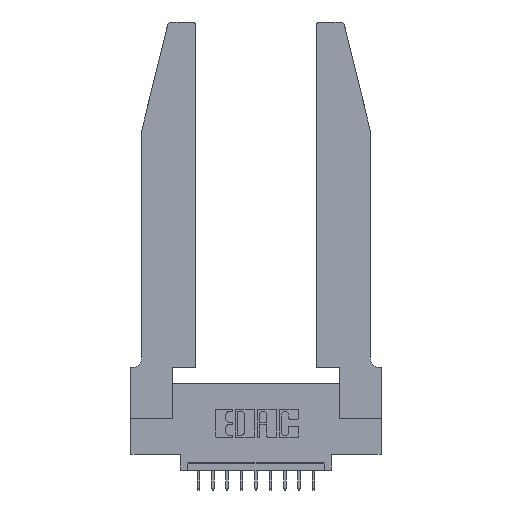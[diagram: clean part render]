
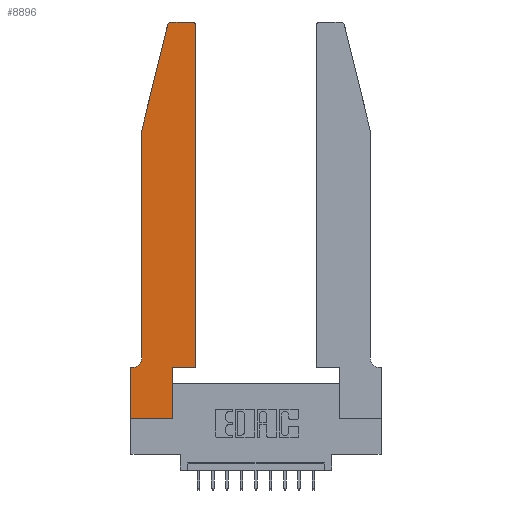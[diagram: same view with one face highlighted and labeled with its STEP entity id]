
A CAD part, top view. The second image highlights one B-rep face of the part: STEP entity #8896.
In plain terms, the highlighted planar face has unit normal (0, 0, 1).
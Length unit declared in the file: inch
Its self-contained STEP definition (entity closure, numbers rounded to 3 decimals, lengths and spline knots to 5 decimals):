
#76 = ORIENTED_EDGE ( 'NONE', *, *, #6097, .T. ) ;
#181 = CARTESIAN_POINT ( 'NONE',  ( 0., 0.35, 0.37 ) ) ;
#246 = EDGE_CURVE ( 'NONE', #8992, #305, #4880, .T. ) ;
#305 = VERTEX_POINT ( 'NONE', #7444 ) ;
#325 = VERTEX_POINT ( 'NONE', #1427 ) ;
#419 = VECTOR ( 'NONE', #12513, 39.37008 ) ;
#554 = CARTESIAN_POINT ( 'NONE',  ( 0.4505, 0.35, 0.37 ) ) ;
#575 = FACE_OUTER_BOUND ( 'NONE', #12629, .T. ) ;
#639 = ORIENTED_EDGE ( 'NONE', *, *, #1111, .T. ) ;
#786 = DIRECTION ( 'NONE',  ( 1., 0., 0. ) ) ;
#902 = VECTOR ( 'NONE', #5218, 39.37008 ) ;
#1111 = EDGE_CURVE ( 'NONE', #7310, #5569, #7624, .T. ) ;
#1407 = PLANE ( 'NONE',  #7855 ) ;
#1427 = CARTESIAN_POINT ( 'NONE',  ( 0., 0., 0.37 ) ) ;
#1849 = CARTESIAN_POINT ( 'NONE',  ( 0.2865, 0., 0.37 ) ) ;
#1931 = VERTEX_POINT ( 'NONE', #10022 ) ;
#2190 = CARTESIAN_POINT ( 'NONE',  ( 0.0755, 2., 0.37 ) ) ;
#2674 = VERTEX_POINT ( 'NONE', #11785 ) ;
#2715 = DIRECTION ( 'NONE',  ( 0., -1., 0. ) ) ;
#2745 = DIRECTION ( 'NONE',  ( 0., 1., 0. ) ) ;
#2868 = VECTOR ( 'NONE', #3057, 39.37008 ) ;
#3057 = DIRECTION ( 'NONE',  ( 0., -1., 0. ) ) ;
#3365 = EDGE_CURVE ( 'NONE', #1931, #7589, #14518, .T. ) ;
#3548 = EDGE_CURVE ( 'NONE', #325, #7310, #7002, .T. ) ;
#3643 = CARTESIAN_POINT ( 'NONE',  ( 0.4505, 0.35, 0.37 ) ) ;
#3966 = VECTOR ( 'NONE', #2715, 39.37008 ) ;
#4075 = DIRECTION ( 'NONE',  ( 1., 0., 0. ) ) ;
#4290 = LINE ( 'NONE', #9312, #2868 ) ;
#4546 = EDGE_CURVE ( 'NONE', #7589, #15937, #14899, .T. ) ;
#4853 = ORIENTED_EDGE ( 'NONE', *, *, #12959, .T. ) ;
#4880 = LINE ( 'NONE', #11265, #3966 ) ;
#5128 = CARTESIAN_POINT ( 'NONE',  ( 0.4505, 0.35, 0.37 ) ) ;
#5218 = DIRECTION ( 'NONE',  ( 0., 1., 0. ) ) ;
#5532 = DIRECTION ( 'NONE',  ( 1., 0., 0. ) ) ;
#5569 = VERTEX_POINT ( 'NONE', #9573 ) ;
#5703 = CARTESIAN_POINT ( 'NONE',  ( 0.0755, 0.35, 0.37 ) ) ;
#5837 = DIRECTION ( 'NONE',  ( -1., 0., 0. ) ) ;
#6079 = ORIENTED_EDGE ( 'NONE', *, *, #4546, .T. ) ;
#6097 = EDGE_CURVE ( 'NONE', #305, #14305, #7039, .T. ) ;
#6785 = DIRECTION ( 'NONE',  ( 0., 0., 1. ) ) ;
#7002 = LINE ( 'NONE', #11985, #11143 ) ;
#7039 = CIRCLE ( 'NONE', #14610, 0.07 ) ;
#7310 = VERTEX_POINT ( 'NONE', #1849 ) ;
#7393 = EDGE_CURVE ( 'NONE', #15937, #2674, #12262, .T. ) ;
#7444 = CARTESIAN_POINT ( 'NONE',  ( 0.0755, 0.42, 0.37 ) ) ;
#7589 = VERTEX_POINT ( 'NONE', #15403 ) ;
#7624 = LINE ( 'NONE', #12599, #902 ) ;
#7855 = AXIS2_PLACEMENT_3D ( 'NONE', #181, #13915, #10490 ) ;
#8086 = EDGE_CURVE ( 'NONE', #14305, #8869, #15975, .T. ) ;
#8372 = CARTESIAN_POINT ( 'NONE',  ( 0.0755, 2., 0.37 ) ) ;
#8452 = VECTOR ( 'NONE', #2745, 39.37008 ) ;
#8549 = CARTESIAN_POINT ( 'NONE',  ( 0.2605, 2.75, 0.37 ) ) ;
#8722 = DIRECTION ( 'NONE',  ( 0., 0., 1. ) ) ;
#8869 = VERTEX_POINT ( 'NONE', #11325 ) ;
#8896 = ADVANCED_FACE ( 'NONE', ( #575 ), #1407, .T. ) ;
#8992 = VERTEX_POINT ( 'NONE', #8372 ) ;
#9017 = CARTESIAN_POINT ( 'NONE',  ( 0.4205, 2.72, 0.37 ) ) ;
#9312 = CARTESIAN_POINT ( 'NONE',  ( 0., 0., 0.37 ) ) ;
#9399 = AXIS2_PLACEMENT_3D ( 'NONE', #13988, #8722, #15151 ) ;
#9573 = CARTESIAN_POINT ( 'NONE',  ( 0.2865, 0.35, 0.37 ) ) ;
#9584 = DIRECTION ( 'NONE',  ( -0.239, -0.971, 0. ) ) ;
#9599 = ORIENTED_EDGE ( 'NONE', *, *, #13100, .T. ) ;
#9758 = DIRECTION ( 'NONE',  ( -1., 0., 0. ) ) ;
#10022 = CARTESIAN_POINT ( 'NONE',  ( 0.4505, 2.72, 0.37 ) ) ;
#10343 = AXIS2_PLACEMENT_3D ( 'NONE', #9017, #6785, #4075 ) ;
#10490 = DIRECTION ( 'NONE',  ( 1., 0., 0. ) ) ;
#11143 = VECTOR ( 'NONE', #786, 39.37008 ) ;
#11265 = CARTESIAN_POINT ( 'NONE',  ( 0.0755, 2., 0.37 ) ) ;
#11325 = CARTESIAN_POINT ( 'NONE',  ( 0., 0.35, 0.37 ) ) ;
#11371 = LINE ( 'NONE', #5128, #8452 ) ;
#11394 = ORIENTED_EDGE ( 'NONE', *, *, #8086, .T. ) ;
#11500 = VECTOR ( 'NONE', #9584, 39.37008 ) ;
#11729 = VECTOR ( 'NONE', #9758, 39.37008 ) ;
#11764 = LINE ( 'NONE', #554, #11771 ) ;
#11771 = VECTOR ( 'NONE', #5532, 39.37008 ) ;
#11785 = CARTESIAN_POINT ( 'NONE',  ( 0.25487, 2.72718, 0.37 ) ) ;
#11985 = CARTESIAN_POINT ( 'NONE',  ( 0., 0., 0.37 ) ) ;
#12053 = DIRECTION ( 'NONE',  ( 0., 0., -1. ) ) ;
#12205 = ORIENTED_EDGE ( 'NONE', *, *, #246, .T. ) ;
#12262 = CIRCLE ( 'NONE', #9399, 0.03 ) ;
#12513 = DIRECTION ( 'NONE',  ( -1., 0., 0. ) ) ;
#12599 = CARTESIAN_POINT ( 'NONE',  ( 0.2865, 0.35, 0.37 ) ) ;
#12629 = EDGE_LOOP ( 'NONE', ( #6079, #14090, #9599, #12205, #76, #11394, #13461, #16173, #639, #4853, #15154, #13911 ) ) ;
#12662 = CARTESIAN_POINT ( 'NONE',  ( 0.284, 2.75, 0.37 ) ) ;
#12959 = EDGE_CURVE ( 'NONE', #5569, #13222, #11764, .T. ) ;
#13100 = EDGE_CURVE ( 'NONE', #2674, #8992, #15707, .T. ) ;
#13222 = VERTEX_POINT ( 'NONE', #3643 ) ;
#13373 = CARTESIAN_POINT ( 'NONE',  ( 0.0055, 0.42, 0.37 ) ) ;
#13454 = EDGE_CURVE ( 'NONE', #8869, #325, #4290, .T. ) ;
#13461 = ORIENTED_EDGE ( 'NONE', *, *, #13454, .T. ) ;
#13911 = ORIENTED_EDGE ( 'NONE', *, *, #3365, .T. ) ;
#13915 = DIRECTION ( 'NONE',  ( 0., 0., 1. ) ) ;
#13988 = CARTESIAN_POINT ( 'NONE',  ( 0.284, 2.72, 0.37 ) ) ;
#14090 = ORIENTED_EDGE ( 'NONE', *, *, #7393, .T. ) ;
#14203 = CARTESIAN_POINT ( 'NONE',  ( 0.0055, 0.35, 0.37 ) ) ;
#14305 = VERTEX_POINT ( 'NONE', #14203 ) ;
#14518 = CIRCLE ( 'NONE', #10343, 0.03 ) ;
#14610 = AXIS2_PLACEMENT_3D ( 'NONE', #13373, #12053, #5837 ) ;
#14899 = LINE ( 'NONE', #8549, #419 ) ;
#15151 = DIRECTION ( 'NONE',  ( 1., 0., 0. ) ) ;
#15154 = ORIENTED_EDGE ( 'NONE', *, *, #15887, .T. ) ;
#15403 = CARTESIAN_POINT ( 'NONE',  ( 0.4205, 2.75, 0.37 ) ) ;
#15707 = LINE ( 'NONE', #2190, #11500 ) ;
#15887 = EDGE_CURVE ( 'NONE', #13222, #1931, #11371, .T. ) ;
#15937 = VERTEX_POINT ( 'NONE', #12662 ) ;
#15975 = LINE ( 'NONE', #5703, #11729 ) ;
#16173 = ORIENTED_EDGE ( 'NONE', *, *, #3548, .T. ) ;
